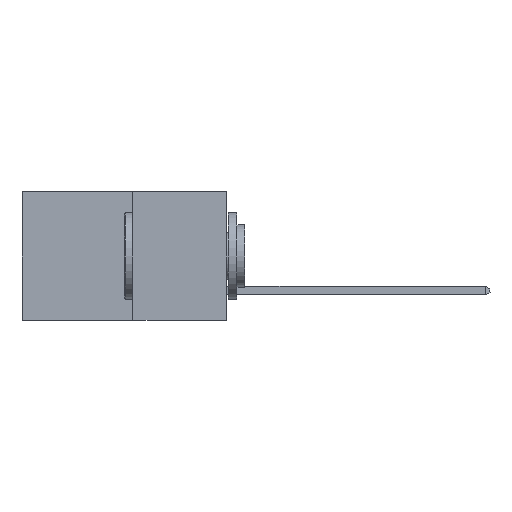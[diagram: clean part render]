
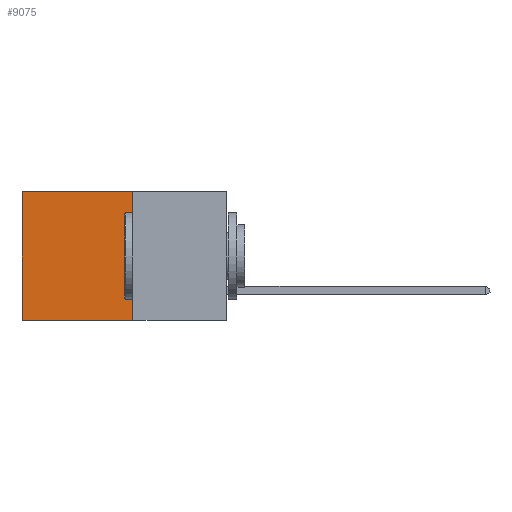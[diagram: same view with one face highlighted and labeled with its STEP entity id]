
A CAD part, left-side view. The second image highlights one B-rep face of the part: STEP entity #9075.
In plain terms, the highlighted planar face has unit normal (-1, 0, 0).
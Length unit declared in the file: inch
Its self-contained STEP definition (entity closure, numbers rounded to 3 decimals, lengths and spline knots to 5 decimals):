
#113 = DIRECTION ( 'NONE',  ( 0., 1., 0. ) ) ;
#246 = VERTEX_POINT ( 'NONE', #11647 ) ;
#426 = CARTESIAN_POINT ( 'NONE',  ( 0.277, 0.27, 0. ) ) ;
#964 = CARTESIAN_POINT ( 'NONE',  ( 0.277, 0.59, 0. ) ) ;
#1088 = DIRECTION ( 'NONE',  ( 0., 1., 0. ) ) ;
#2058 = ORIENTED_EDGE ( 'NONE', *, *, #8793, .T. ) ;
#2584 = AXIS2_PLACEMENT_3D ( 'NONE', #6391, #4196, #11645 ) ;
#2802 = ORIENTED_EDGE ( 'NONE', *, *, #9078, .T. ) ;
#3271 = VERTEX_POINT ( 'NONE', #426 ) ;
#4005 = LINE ( 'NONE', #10910, #12146 ) ;
#4196 = DIRECTION ( 'NONE',  ( 1., 0., 0. ) ) ;
#4794 = EDGE_LOOP ( 'NONE', ( #2802, #8800, #9439, #2058 ) ) ;
#4961 = LINE ( 'NONE', #7830, #9931 ) ;
#5014 = FACE_OUTER_BOUND ( 'NONE', #4794, .T. ) ;
#5533 = EDGE_CURVE ( 'NONE', #3271, #7061, #4961, .T. ) ;
#6138 = CARTESIAN_POINT ( 'NONE',  ( 0.277, 0.27, -0.37 ) ) ;
#6244 = LINE ( 'NONE', #9076, #11462 ) ;
#6391 = CARTESIAN_POINT ( 'NONE',  ( 0.277, 0.27, -0.37 ) ) ;
#6470 = VERTEX_POINT ( 'NONE', #964 ) ;
#7061 = VERTEX_POINT ( 'NONE', #6138 ) ;
#7491 = DIRECTION ( 'NONE',  ( 0., 0., -1. ) ) ;
#7830 = CARTESIAN_POINT ( 'NONE',  ( 0.277, 0.27, -0.37 ) ) ;
#8280 = DIRECTION ( 'NONE',  ( 0., 0., -1. ) ) ;
#8793 = EDGE_CURVE ( 'NONE', #3271, #6470, #6244, .T. ) ;
#8800 = ORIENTED_EDGE ( 'NONE', *, *, #12890, .F. ) ;
#9075 = ADVANCED_FACE ( 'NONE', ( #5014 ), #10613, .F. ) ;
#9076 = CARTESIAN_POINT ( 'NONE',  ( 0.277, 0.27, 0. ) ) ;
#9078 = EDGE_CURVE ( 'NONE', #6470, #246, #13008, .T. ) ;
#9439 = ORIENTED_EDGE ( 'NONE', *, *, #5533, .F. ) ;
#9931 = VECTOR ( 'NONE', #8280, 39.37008 ) ;
#10613 = PLANE ( 'NONE',  #2584 ) ;
#10650 = VECTOR ( 'NONE', #7491, 39.37008 ) ;
#10910 = CARTESIAN_POINT ( 'NONE',  ( 0.277, 0.27, -0.37 ) ) ;
#11462 = VECTOR ( 'NONE', #113, 39.37008 ) ;
#11645 = DIRECTION ( 'NONE',  ( 0., 0., -1. ) ) ;
#11647 = CARTESIAN_POINT ( 'NONE',  ( 0.277, 0.59, -0.37 ) ) ;
#12146 = VECTOR ( 'NONE', #1088, 39.37008 ) ;
#12890 = EDGE_CURVE ( 'NONE', #7061, #246, #4005, .T. ) ;
#13008 = LINE ( 'NONE', #13615, #10650 ) ;
#13615 = CARTESIAN_POINT ( 'NONE',  ( 0.277, 0.59, -0.37 ) ) ;
